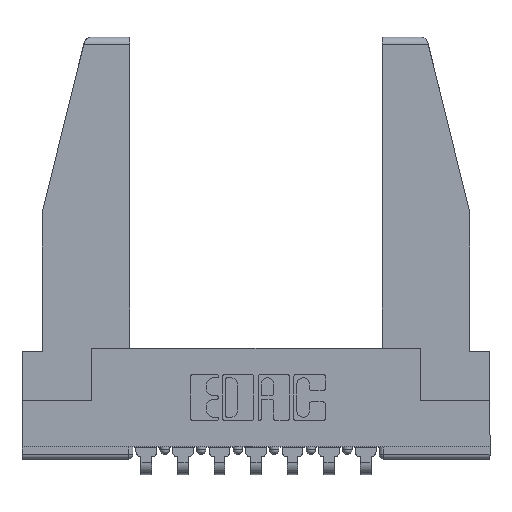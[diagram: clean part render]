
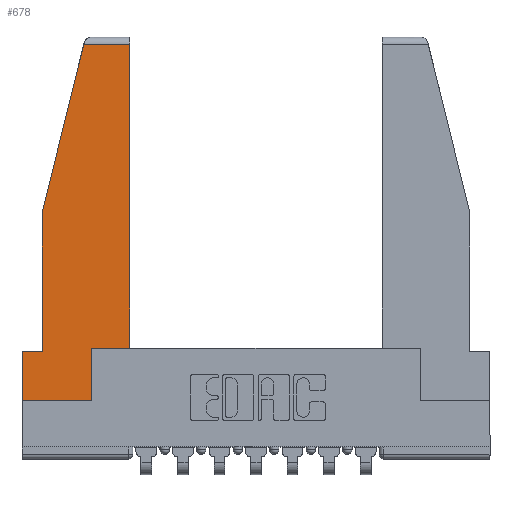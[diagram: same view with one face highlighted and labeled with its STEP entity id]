
A CAD part, top view. The second image highlights one B-rep face of the part: STEP entity #678.
In plain terms, the highlighted planar face has unit normal (0, 0, 1).
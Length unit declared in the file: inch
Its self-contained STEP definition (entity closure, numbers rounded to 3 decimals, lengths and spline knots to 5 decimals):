
#221 = ORIENTED_EDGE ( 'NONE', *, *, #6397, .T. ) ;
#380 = LINE ( 'NONE', #4550, #2817 ) ;
#427 = AXIS2_PLACEMENT_3D ( 'NONE', #9382, #4426, #11334 ) ;
#678 = ADVANCED_FACE ( 'NONE', ( #4667 ), #8670, .T. ) ;
#743 = LINE ( 'NONE', #3738, #10585 ) ;
#943 = CARTESIAN_POINT ( 'NONE',  ( 0.461, 0.223, 0. ) ) ;
#1056 = EDGE_CURVE ( 'NONE', #1933, #3142, #1409, .T. ) ;
#1085 = DIRECTION ( 'NONE',  ( 0., -1., 0. ) ) ;
#1300 = EDGE_CURVE ( 'NONE', #5910, #6845, #9342, .T. ) ;
#1409 = LINE ( 'NONE', #11324, #7346 ) ;
#1933 = VERTEX_POINT ( 'NONE', #7421 ) ;
#2540 = EDGE_CURVE ( 'NONE', #3717, #6468, #743, .T. ) ;
#2691 = VECTOR ( 'NONE', #3877, 39.37008 ) ;
#2751 = EDGE_LOOP ( 'NONE', ( #3330, #10672, #7362, #6482, #6185, #221, #5525, #11686, #6771 ) ) ;
#2784 = CARTESIAN_POINT ( 'NONE',  ( 0.297, 0.223, 0. ) ) ;
#2817 = VECTOR ( 'NONE', #4482, 39.37008 ) ;
#2922 = CARTESIAN_POINT ( 'NONE',  ( 0.297, 0., 0. ) ) ;
#3022 = CARTESIAN_POINT ( 'NONE',  ( 0., 0.21, 0. ) ) ;
#3048 = LINE ( 'NONE', #2922, #3933 ) ;
#3088 = LINE ( 'NONE', #3022, #7859 ) ;
#3142 = VERTEX_POINT ( 'NONE', #6506 ) ;
#3330 = ORIENTED_EDGE ( 'NONE', *, *, #2540, .T. ) ;
#3676 = CARTESIAN_POINT ( 'NONE',  ( 0., 0.21, 0. ) ) ;
#3717 = VERTEX_POINT ( 'NONE', #943 ) ;
#3738 = CARTESIAN_POINT ( 'NONE',  ( 0.461, 0.223, 0. ) ) ;
#3785 = CARTESIAN_POINT ( 'NONE',  ( 0., 1.52, 0. ) ) ;
#3877 = DIRECTION ( 'NONE',  ( -1., 0., 0. ) ) ;
#3897 = VERTEX_POINT ( 'NONE', #7066 ) ;
#3933 = VECTOR ( 'NONE', #4830, 39.37008 ) ;
#4426 = DIRECTION ( 'NONE',  ( 0., 0., 1. ) ) ;
#4482 = DIRECTION ( 'NONE',  ( 1., 0., 0. ) ) ;
#4550 = CARTESIAN_POINT ( 'NONE',  ( 0.297, 0.223, 0. ) ) ;
#4667 = FACE_OUTER_BOUND ( 'NONE', #2751, .T. ) ;
#4830 = DIRECTION ( 'NONE',  ( 0., 1., 0. ) ) ;
#4929 = VECTOR ( 'NONE', #10720, 39.37008 ) ;
#4963 = LINE ( 'NONE', #3785, #4929 ) ;
#5001 = DIRECTION ( 'NONE',  ( 0., -1., 0. ) ) ;
#5383 = CARTESIAN_POINT ( 'NONE',  ( 0., 0.21, 0. ) ) ;
#5397 = EDGE_CURVE ( 'NONE', #6468, #5910, #4963, .T. ) ;
#5525 = ORIENTED_EDGE ( 'NONE', *, *, #1056, .T. ) ;
#5910 = VERTEX_POINT ( 'NONE', #12640 ) ;
#5957 = CARTESIAN_POINT ( 'NONE',  ( 0.271, 1.55, 0. ) ) ;
#6050 = EDGE_CURVE ( 'NONE', #7163, #3717, #380, .T. ) ;
#6185 = ORIENTED_EDGE ( 'NONE', *, *, #12004, .T. ) ;
#6397 = EDGE_CURVE ( 'NONE', #10813, #1933, #3088, .T. ) ;
#6468 = VERTEX_POINT ( 'NONE', #11256 ) ;
#6482 = ORIENTED_EDGE ( 'NONE', *, *, #9278, .T. ) ;
#6506 = CARTESIAN_POINT ( 'NONE',  ( 0.297, 0., 0. ) ) ;
#6751 = LINE ( 'NONE', #3676, #2691 ) ;
#6771 = ORIENTED_EDGE ( 'NONE', *, *, #6050, .T. ) ;
#6845 = VERTEX_POINT ( 'NONE', #11166 ) ;
#6889 = DIRECTION ( 'NONE',  ( 0., 1., 0. ) ) ;
#7066 = CARTESIAN_POINT ( 'NONE',  ( 0.086, 0.21, 0. ) ) ;
#7163 = VERTEX_POINT ( 'NONE', #2784 ) ;
#7276 = VECTOR ( 'NONE', #5001, 39.37008 ) ;
#7346 = VECTOR ( 'NONE', #11566, 39.37008 ) ;
#7362 = ORIENTED_EDGE ( 'NONE', *, *, #1300, .T. ) ;
#7421 = CARTESIAN_POINT ( 'NONE',  ( 0., 0., 0. ) ) ;
#7859 = VECTOR ( 'NONE', #1085, 39.37008 ) ;
#7991 = DIRECTION ( 'NONE',  ( -0.239, -0.971, 0. ) ) ;
#8670 = PLANE ( 'NONE',  #427 ) ;
#8955 = EDGE_CURVE ( 'NONE', #3142, #7163, #3048, .T. ) ;
#9278 = EDGE_CURVE ( 'NONE', #6845, #3897, #11801, .T. ) ;
#9342 = LINE ( 'NONE', #5957, #11375 ) ;
#9382 = CARTESIAN_POINT ( 'NONE',  ( 0., 0., 0. ) ) ;
#10585 = VECTOR ( 'NONE', #6889, 39.37008 ) ;
#10672 = ORIENTED_EDGE ( 'NONE', *, *, #5397, .T. ) ;
#10720 = DIRECTION ( 'NONE',  ( -1., 0., 0. ) ) ;
#10813 = VERTEX_POINT ( 'NONE', #5383 ) ;
#11166 = CARTESIAN_POINT ( 'NONE',  ( 0.086, 0.8, 0. ) ) ;
#11256 = CARTESIAN_POINT ( 'NONE',  ( 0.461, 1.52, 0. ) ) ;
#11324 = CARTESIAN_POINT ( 'NONE',  ( 0., 0., 0. ) ) ;
#11334 = DIRECTION ( 'NONE',  ( 1., 0., 0. ) ) ;
#11375 = VECTOR ( 'NONE', #7991, 39.37008 ) ;
#11566 = DIRECTION ( 'NONE',  ( 1., 0., 0. ) ) ;
#11686 = ORIENTED_EDGE ( 'NONE', *, *, #8955, .T. ) ;
#11801 = LINE ( 'NONE', #12764, #7276 ) ;
#12004 = EDGE_CURVE ( 'NONE', #3897, #10813, #6751, .T. ) ;
#12640 = CARTESIAN_POINT ( 'NONE',  ( 0.2636, 1.52, 0. ) ) ;
#12764 = CARTESIAN_POINT ( 'NONE',  ( 0.086, 0.8, 0. ) ) ;
